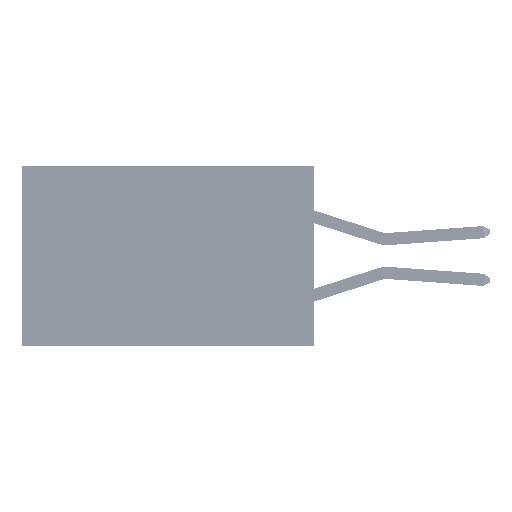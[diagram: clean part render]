
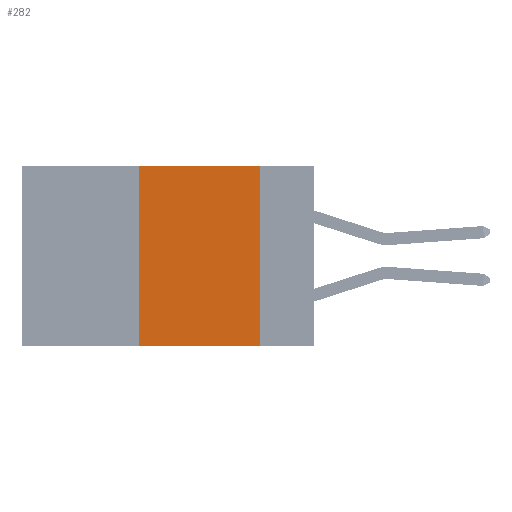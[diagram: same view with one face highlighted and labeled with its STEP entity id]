
A CAD part, left-side view. The second image highlights one B-rep face of the part: STEP entity #282.
In plain terms, the highlighted planar face has unit normal (-1, 0, 0).
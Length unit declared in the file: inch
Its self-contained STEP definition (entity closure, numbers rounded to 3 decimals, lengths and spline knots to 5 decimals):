
#282 = ADVANCED_FACE ( 'NONE', ( #26669 ), #29642, .F. ) ;
#1879 = VERTEX_POINT ( 'NONE', #17284 ) ;
#2139 = DIRECTION ( 'NONE',  ( 0., 0., -1. ) ) ;
#2469 = EDGE_CURVE ( 'NONE', #18085, #42158, #31216, .T. ) ;
#3637 = VECTOR ( 'NONE', #2139, 39.37008 ) ;
#4234 = AXIS2_PLACEMENT_3D ( 'NONE', #6179, #9472, #41284 ) ;
#4568 = CARTESIAN_POINT ( 'NONE',  ( 0., 0.36, 0. ) ) ;
#6179 = CARTESIAN_POINT ( 'NONE',  ( 0., 0.6, 0. ) ) ;
#6567 = CARTESIAN_POINT ( 'NONE',  ( 0., 0.11, 0. ) ) ;
#8059 = ORIENTED_EDGE ( 'NONE', *, *, #2469, .F. ) ;
#9472 = DIRECTION ( 'NONE',  ( 1., 0., 0. ) ) ;
#10026 = VECTOR ( 'NONE', #14105, 39.37008 ) ;
#14105 = DIRECTION ( 'NONE',  ( 0., -1., 0. ) ) ;
#17284 = CARTESIAN_POINT ( 'NONE',  ( 0., 0.36, -0.37 ) ) ;
#18085 = VERTEX_POINT ( 'NONE', #43184 ) ;
#21855 = LINE ( 'NONE', #23302, #28567 ) ;
#22629 = DIRECTION ( 'NONE',  ( 0., 0., 1. ) ) ;
#23302 = CARTESIAN_POINT ( 'NONE',  ( 0., 0.36, 0. ) ) ;
#26669 = FACE_OUTER_BOUND ( 'NONE', #27605, .T. ) ;
#26885 = CARTESIAN_POINT ( 'NONE',  ( 0., 0.6, 0. ) ) ;
#27605 = EDGE_LOOP ( 'NONE', ( #8059, #32862, #41796, #30077 ) ) ;
#28567 = VECTOR ( 'NONE', #22629, 39.37008 ) ;
#28830 = VECTOR ( 'NONE', #46428, 39.37008 ) ;
#28885 = EDGE_CURVE ( 'NONE', #1879, #48111, #21855, .T. ) ;
#29642 = PLANE ( 'NONE',  #4234 ) ;
#30077 = ORIENTED_EDGE ( 'NONE', *, *, #43355, .T. ) ;
#31216 = LINE ( 'NONE', #6567, #3637 ) ;
#32862 = ORIENTED_EDGE ( 'NONE', *, *, #45041, .F. ) ;
#33222 = CARTESIAN_POINT ( 'NONE',  ( 0., 0.11, -0.37 ) ) ;
#35746 = LINE ( 'NONE', #41423, #10026 ) ;
#41284 = DIRECTION ( 'NONE',  ( 0., 0., -1. ) ) ;
#41423 = CARTESIAN_POINT ( 'NONE',  ( 0., 0.6, -0.37 ) ) ;
#41796 = ORIENTED_EDGE ( 'NONE', *, *, #28885, .F. ) ;
#42158 = VERTEX_POINT ( 'NONE', #33222 ) ;
#43184 = CARTESIAN_POINT ( 'NONE',  ( 0., 0.11, 0. ) ) ;
#43355 = EDGE_CURVE ( 'NONE', #1879, #42158, #35746, .T. ) ;
#45041 = EDGE_CURVE ( 'NONE', #48111, #18085, #50257, .T. ) ;
#46428 = DIRECTION ( 'NONE',  ( 0., -1., 0. ) ) ;
#48111 = VERTEX_POINT ( 'NONE', #4568 ) ;
#50257 = LINE ( 'NONE', #26885, #28830 ) ;
